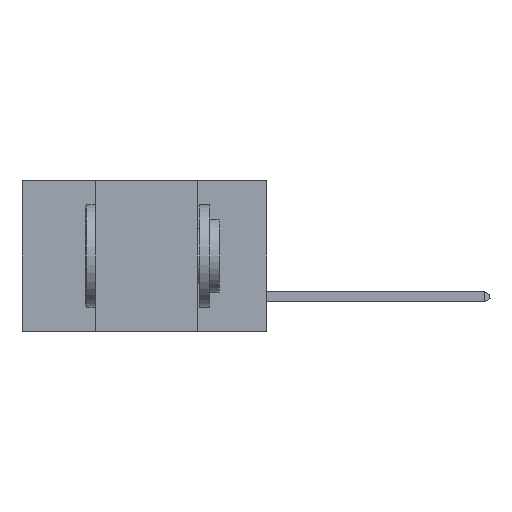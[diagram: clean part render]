
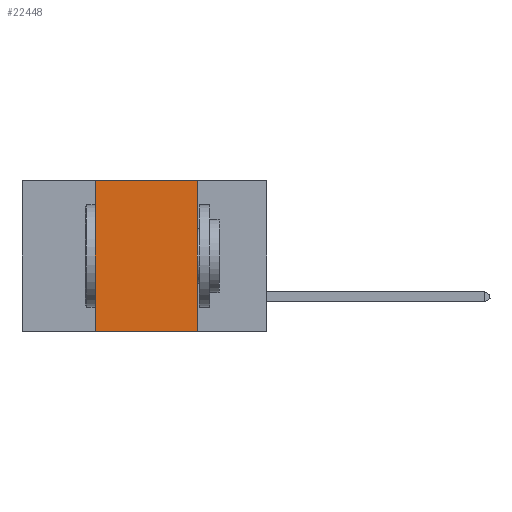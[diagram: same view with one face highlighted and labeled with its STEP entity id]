
A CAD part, left-side view. The second image highlights one B-rep face of the part: STEP entity #22448.
In plain terms, the highlighted planar face has unit normal (-1, 0, 0).
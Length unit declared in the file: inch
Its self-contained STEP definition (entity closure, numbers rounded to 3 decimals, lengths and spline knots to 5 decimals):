
#328 = CARTESIAN_POINT ( 'NONE',  ( 0., 0.17, -0.37 ) ) ;
#1060 = LINE ( 'NONE', #29593, #8016 ) ;
#1212 = CARTESIAN_POINT ( 'NONE',  ( 0., 0.6, 0. ) ) ;
#2504 = EDGE_LOOP ( 'NONE', ( #17587, #5676, #2819, #13084 ) ) ;
#2819 = ORIENTED_EDGE ( 'NONE', *, *, #20930, .F. ) ;
#2999 = CARTESIAN_POINT ( 'NONE',  ( 0., 0.42, 0. ) ) ;
#3668 = DIRECTION ( 'NONE',  ( 0., 0., -1. ) ) ;
#3802 = DIRECTION ( 'NONE',  ( 0., 0., -1. ) ) ;
#5676 = ORIENTED_EDGE ( 'NONE', *, *, #15130, .F. ) ;
#5905 = VERTEX_POINT ( 'NONE', #328 ) ;
#6752 = LINE ( 'NONE', #2999, #19922 ) ;
#8016 = VECTOR ( 'NONE', #24469, 39.37008 ) ;
#8215 = VERTEX_POINT ( 'NONE', #33333 ) ;
#9728 = EDGE_CURVE ( 'NONE', #22786, #5905, #31760, .T. ) ;
#11132 = VECTOR ( 'NONE', #18065, 39.37008 ) ;
#13084 = ORIENTED_EDGE ( 'NONE', *, *, #9728, .T. ) ;
#14232 = CARTESIAN_POINT ( 'NONE',  ( 0., 0.42, 0. ) ) ;
#15130 = EDGE_CURVE ( 'NONE', #18327, #8215, #1060, .T. ) ;
#15739 = CARTESIAN_POINT ( 'NONE',  ( 0., 0.42, -0.37 ) ) ;
#16041 = VECTOR ( 'NONE', #3668, 39.37008 ) ;
#17587 = ORIENTED_EDGE ( 'NONE', *, *, #29506, .F. ) ;
#18065 = DIRECTION ( 'NONE',  ( 0., -1., 0. ) ) ;
#18327 = VERTEX_POINT ( 'NONE', #14232 ) ;
#19567 = DIRECTION ( 'NONE',  ( 1., 0., 0. ) ) ;
#19922 = VECTOR ( 'NONE', #29101, 39.37008 ) ;
#20687 = CARTESIAN_POINT ( 'NONE',  ( 0., 0.6, -0.37 ) ) ;
#20930 = EDGE_CURVE ( 'NONE', #22786, #18327, #6752, .T. ) ;
#22448 = ADVANCED_FACE ( 'NONE', ( #25087 ), #32109, .F. ) ;
#22786 = VERTEX_POINT ( 'NONE', #15739 ) ;
#22960 = LINE ( 'NONE', #24509, #16041 ) ;
#24469 = DIRECTION ( 'NONE',  ( 0., -1., 0. ) ) ;
#24509 = CARTESIAN_POINT ( 'NONE',  ( 0., 0.17, 0. ) ) ;
#25087 = FACE_OUTER_BOUND ( 'NONE', #2504, .T. ) ;
#29101 = DIRECTION ( 'NONE',  ( 0., 0., 1. ) ) ;
#29506 = EDGE_CURVE ( 'NONE', #8215, #5905, #22960, .T. ) ;
#29593 = CARTESIAN_POINT ( 'NONE',  ( 0., 0.6, 0. ) ) ;
#31437 = AXIS2_PLACEMENT_3D ( 'NONE', #1212, #19567, #3802 ) ;
#31760 = LINE ( 'NONE', #20687, #11132 ) ;
#32109 = PLANE ( 'NONE',  #31437 ) ;
#33333 = CARTESIAN_POINT ( 'NONE',  ( 0., 0.17, 0. ) ) ;
